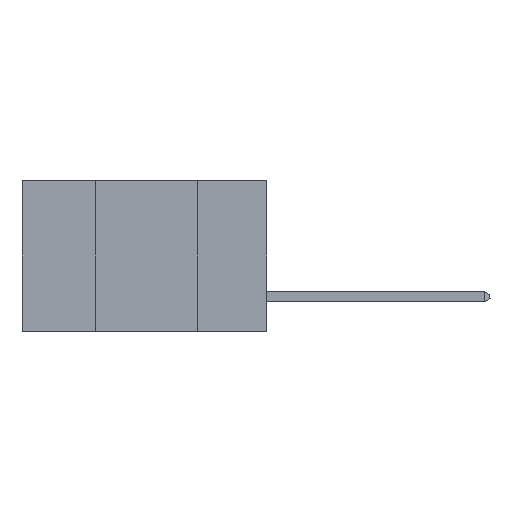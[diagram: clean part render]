
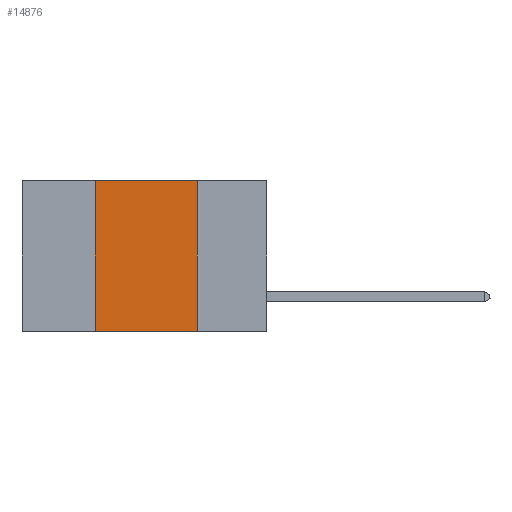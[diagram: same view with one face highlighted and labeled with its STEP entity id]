
A CAD part, left-side view. The second image highlights one B-rep face of the part: STEP entity #14876.
In plain terms, the highlighted planar face has unit normal (-1, 0, 0).
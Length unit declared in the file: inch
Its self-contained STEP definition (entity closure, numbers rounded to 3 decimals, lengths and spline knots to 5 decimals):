
#643 = VECTOR ( 'NONE', #3505, 39.37008 ) ;
#949 = ORIENTED_EDGE ( 'NONE', *, *, #11257, .F. ) ;
#1415 = LINE ( 'NONE', #15264, #643 ) ;
#1946 = CARTESIAN_POINT ( 'NONE',  ( 0., 0.17, -0.37 ) ) ;
#3505 = DIRECTION ( 'NONE',  ( 0., -1., 0. ) ) ;
#3543 = VECTOR ( 'NONE', #20830, 39.37008 ) ;
#3676 = DIRECTION ( 'NONE',  ( 1., 0., 0. ) ) ;
#3864 = DIRECTION ( 'NONE',  ( 0., -1., 0. ) ) ;
#4247 = CARTESIAN_POINT ( 'NONE',  ( 0., 0.17, 0. ) ) ;
#4300 = VERTEX_POINT ( 'NONE', #1946 ) ;
#4576 = VECTOR ( 'NONE', #15695, 39.37008 ) ;
#4985 = AXIS2_PLACEMENT_3D ( 'NONE', #29475, #3676, #20241 ) ;
#6685 = VECTOR ( 'NONE', #3864, 39.37008 ) ;
#7827 = VERTEX_POINT ( 'NONE', #15204 ) ;
#8529 = CARTESIAN_POINT ( 'NONE',  ( 0., 0.42, 0. ) ) ;
#8546 = EDGE_CURVE ( 'NONE', #17361, #18646, #1415, .T. ) ;
#8756 = ORIENTED_EDGE ( 'NONE', *, *, #29198, .F. ) ;
#9481 = ORIENTED_EDGE ( 'NONE', *, *, #8546, .F. ) ;
#10841 = LINE ( 'NONE', #8529, #4576 ) ;
#11257 = EDGE_CURVE ( 'NONE', #18646, #4300, #28566, .T. ) ;
#13222 = CARTESIAN_POINT ( 'NONE',  ( 0., 0.6, -0.37 ) ) ;
#14876 = ADVANCED_FACE ( 'NONE', ( #22969 ), #22505, .F. ) ;
#15204 = CARTESIAN_POINT ( 'NONE',  ( 0., 0.42, -0.37 ) ) ;
#15264 = CARTESIAN_POINT ( 'NONE',  ( 0., 0.6, 0. ) ) ;
#15695 = DIRECTION ( 'NONE',  ( 0., 0., 1. ) ) ;
#17361 = VERTEX_POINT ( 'NONE', #26843 ) ;
#17879 = LINE ( 'NONE', #13222, #6685 ) ;
#18480 = EDGE_CURVE ( 'NONE', #7827, #4300, #17879, .T. ) ;
#18646 = VERTEX_POINT ( 'NONE', #21037 ) ;
#20241 = DIRECTION ( 'NONE',  ( 0., 0., -1. ) ) ;
#20830 = DIRECTION ( 'NONE',  ( 0., 0., -1. ) ) ;
#21037 = CARTESIAN_POINT ( 'NONE',  ( 0., 0.17, 0. ) ) ;
#22505 = PLANE ( 'NONE',  #4985 ) ;
#22969 = FACE_OUTER_BOUND ( 'NONE', #23037, .T. ) ;
#23037 = EDGE_LOOP ( 'NONE', ( #949, #9481, #8756, #28418 ) ) ;
#26843 = CARTESIAN_POINT ( 'NONE',  ( 0., 0.42, 0. ) ) ;
#28418 = ORIENTED_EDGE ( 'NONE', *, *, #18480, .T. ) ;
#28566 = LINE ( 'NONE', #4247, #3543 ) ;
#29198 = EDGE_CURVE ( 'NONE', #7827, #17361, #10841, .T. ) ;
#29475 = CARTESIAN_POINT ( 'NONE',  ( 0., 0.6, 0. ) ) ;
